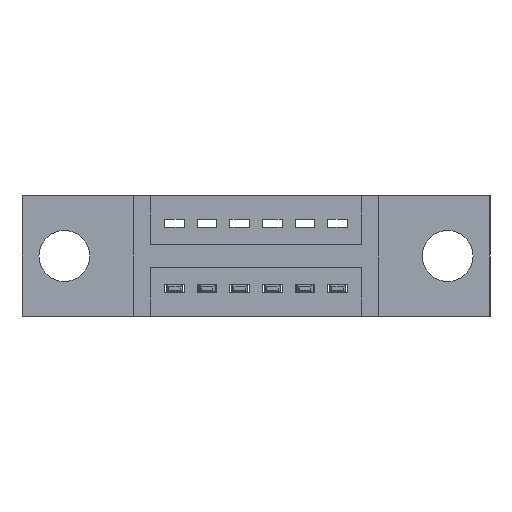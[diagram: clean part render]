
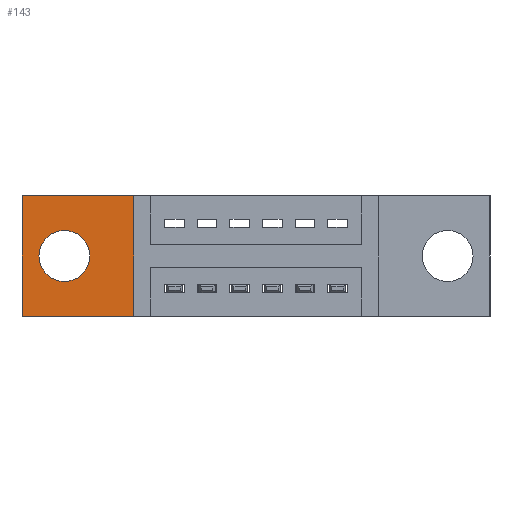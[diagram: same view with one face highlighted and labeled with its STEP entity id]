
A CAD part, front view. The second image highlights one B-rep face of the part: STEP entity #143.
In plain terms, the highlighted planar face has unit normal (0, -1, 0).
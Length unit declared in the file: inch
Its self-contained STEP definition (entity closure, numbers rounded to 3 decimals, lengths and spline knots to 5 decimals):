
#113 = CARTESIAN_POINT ( 'NONE',  ( 0., 0.17, -0.37 ) ) ;
#143 = ADVANCED_FACE ( 'NONE', ( #6873, #7528 ), #3197, .T. ) ;
#315 = EDGE_CURVE ( 'NONE', #5867, #6211, #6755, .T. ) ;
#469 = CARTESIAN_POINT ( 'NONE',  ( 0.13, 0.17, -0.185 ) ) ;
#647 = DIRECTION ( 'NONE',  ( 1., 0., 0. ) ) ;
#653 = AXIS2_PLACEMENT_3D ( 'NONE', #6564, #3015, #8599 ) ;
#671 = LINE ( 'NONE', #2183, #3045 ) ;
#1965 = CARTESIAN_POINT ( 'NONE',  ( 0., 0.17, -0.37 ) ) ;
#2135 = CARTESIAN_POINT ( 'NONE',  ( 0.13, 0.17, -0.263 ) ) ;
#2180 = AXIS2_PLACEMENT_3D ( 'NONE', #1965, #7059, #3640 ) ;
#2183 = CARTESIAN_POINT ( 'NONE',  ( 0., 0.17, 0. ) ) ;
#2600 = EDGE_LOOP ( 'NONE', ( #7360, #8910, #6910, #5739 ) ) ;
#2721 = VECTOR ( 'NONE', #647, 39.37008 ) ;
#2919 = DIRECTION ( 'NONE',  ( 0., 0., -1. ) ) ;
#3015 = DIRECTION ( 'NONE',  ( 0., -1., 0. ) ) ;
#3033 = CARTESIAN_POINT ( 'NONE',  ( 0., 0.17, 0. ) ) ;
#3045 = VECTOR ( 'NONE', #2919, 39.37008 ) ;
#3197 = PLANE ( 'NONE',  #2180 ) ;
#3242 = AXIS2_PLACEMENT_3D ( 'NONE', #469, #9059, #8332 ) ;
#3640 = DIRECTION ( 'NONE',  ( 0., 0., -1. ) ) ;
#3697 = CARTESIAN_POINT ( 'NONE',  ( 0.3425, 0.17, 0. ) ) ;
#4135 = EDGE_CURVE ( 'NONE', #6211, #5867, #5911, .T. ) ;
#4317 = VERTEX_POINT ( 'NONE', #113 ) ;
#4332 = EDGE_CURVE ( 'NONE', #7458, #6008, #6143, .T. ) ;
#5218 = VERTEX_POINT ( 'NONE', #3033 ) ;
#5446 = ORIENTED_EDGE ( 'NONE', *, *, #4135, .F. ) ;
#5739 = ORIENTED_EDGE ( 'NONE', *, *, #8085, .T. ) ;
#5867 = VERTEX_POINT ( 'NONE', #7812 ) ;
#5887 = DIRECTION ( 'NONE',  ( 0., 0., 1. ) ) ;
#5911 = CIRCLE ( 'NONE', #653, 0.078 ) ;
#6008 = VERTEX_POINT ( 'NONE', #7640 ) ;
#6088 = CARTESIAN_POINT ( 'NONE',  ( 0., 0.17, 0. ) ) ;
#6102 = CARTESIAN_POINT ( 'NONE',  ( 0., 0.17, -0.37 ) ) ;
#6143 = LINE ( 'NONE', #3697, #8260 ) ;
#6203 = ORIENTED_EDGE ( 'NONE', *, *, #315, .F. ) ;
#6211 = VERTEX_POINT ( 'NONE', #2135 ) ;
#6353 = LINE ( 'NONE', #6088, #7800 ) ;
#6564 = CARTESIAN_POINT ( 'NONE',  ( 0.13, 0.17, -0.185 ) ) ;
#6755 = CIRCLE ( 'NONE', #3242, 0.078 ) ;
#6856 = EDGE_CURVE ( 'NONE', #5218, #4317, #671, .T. ) ;
#6859 = EDGE_LOOP ( 'NONE', ( #6203, #5446 ) ) ;
#6873 = FACE_BOUND ( 'NONE', #6859, .T. ) ;
#6910 = ORIENTED_EDGE ( 'NONE', *, *, #4332, .T. ) ;
#7059 = DIRECTION ( 'NONE',  ( 0., -1., 0. ) ) ;
#7318 = CARTESIAN_POINT ( 'NONE',  ( 0.3425, 0.17, -0.37 ) ) ;
#7360 = ORIENTED_EDGE ( 'NONE', *, *, #6856, .T. ) ;
#7458 = VERTEX_POINT ( 'NONE', #7318 ) ;
#7528 = FACE_OUTER_BOUND ( 'NONE', #2600, .T. ) ;
#7550 = DIRECTION ( 'NONE',  ( -1., 0., 0. ) ) ;
#7640 = CARTESIAN_POINT ( 'NONE',  ( 0.3425, 0.17, 0. ) ) ;
#7800 = VECTOR ( 'NONE', #7550, 39.37008 ) ;
#7812 = CARTESIAN_POINT ( 'NONE',  ( 0.13, 0.17, -0.107 ) ) ;
#8085 = EDGE_CURVE ( 'NONE', #6008, #5218, #6353, .T. ) ;
#8129 = LINE ( 'NONE', #6102, #2721 ) ;
#8260 = VECTOR ( 'NONE', #5887, 39.37008 ) ;
#8332 = DIRECTION ( 'NONE',  ( 0., 0., -1. ) ) ;
#8599 = DIRECTION ( 'NONE',  ( 0., 0., -1. ) ) ;
#8857 = EDGE_CURVE ( 'NONE', #4317, #7458, #8129, .T. ) ;
#8910 = ORIENTED_EDGE ( 'NONE', *, *, #8857, .T. ) ;
#9059 = DIRECTION ( 'NONE',  ( 0., -1., 0. ) ) ;
